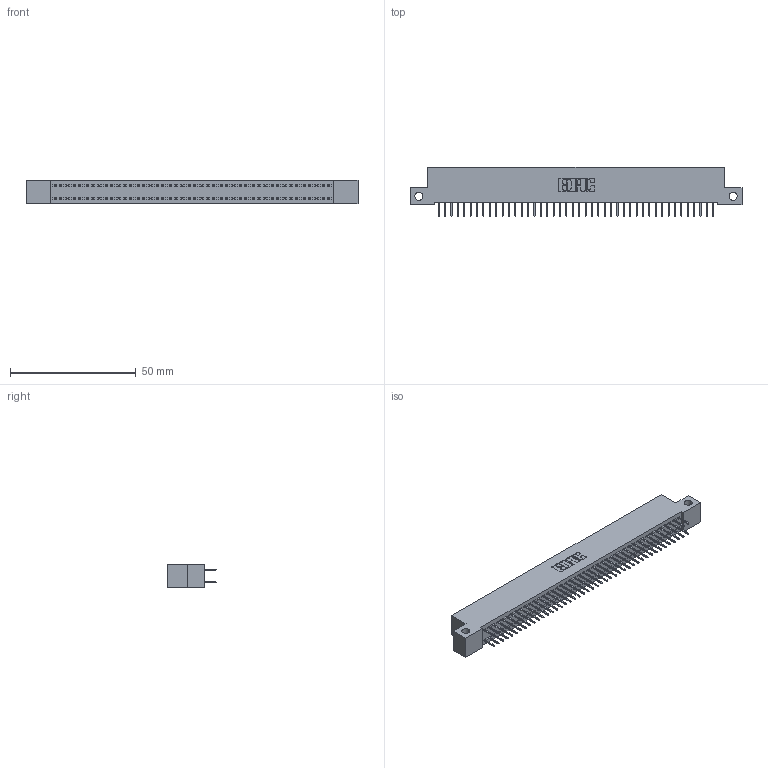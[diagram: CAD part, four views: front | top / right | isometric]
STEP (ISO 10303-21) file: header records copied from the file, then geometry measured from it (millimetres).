
FILE_DESCRIPTION (( 'STEP AP203' ), '1' );
FILE_NAME ('342-088-524-212.STEP', '2018-08-13T20:28:02', ( '' ), ( '' ), 'SwSTEP 2.0', 'SolidWorks 2016', '' );
FILE_SCHEMA (( 'CONFIG_CONTROL_DESIGN' ));
Length unit declared in the file: inch
Products named in the file (3): 342 Part_Side Mount; 345-292-001_345-293-124; 342-088-524-212
Assembly tree (89 placements, depth 2):
  342-088-524-212
    342 Part_Side Mount
    345-292-001_345-293-124  x88
Bounding box: 132.08 x 19.69 x 9.4 mm (x, y, z)
Volume: 11669.7 mm3; surface area: 18538.5 mm2
Topology: 89 solids, 89 shells, 5038 faces, 14291 edges, 9174 vertices
Faces by surface type: plane 3762, cylinder 1276
Entity records: 27993 total; most frequent: CARTESIAN_POINT 4634, ORIENTED_EDGE 4570, DIRECTION 3957, EDGE_CURVE 2285, LINE 2161, VECTOR 2161, VERTEX_POINT 1518, AXIS2_PLACEMENT_3D 898
